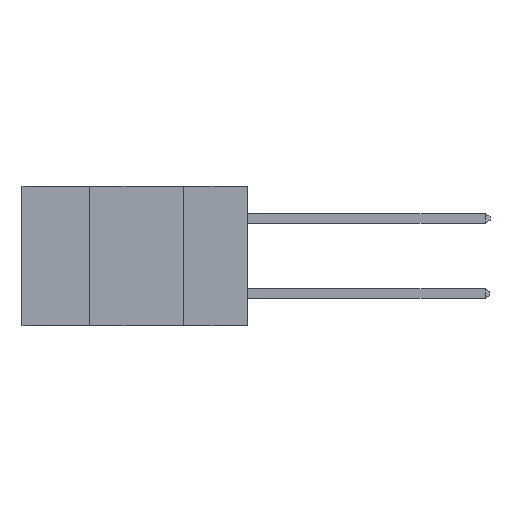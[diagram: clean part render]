
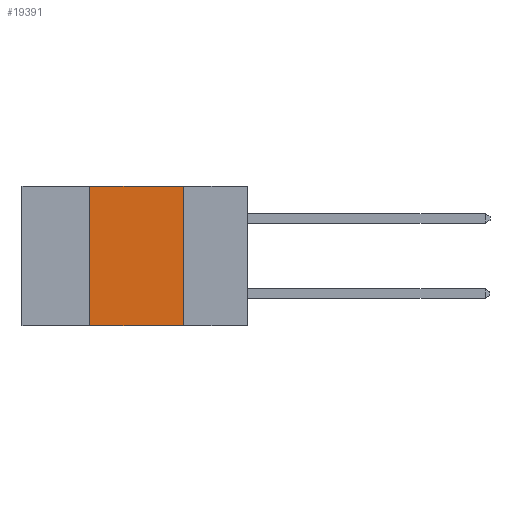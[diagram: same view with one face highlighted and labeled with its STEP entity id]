
A CAD part, left-side view. The second image highlights one B-rep face of the part: STEP entity #19391.
In plain terms, the highlighted planar face has unit normal (-1, 0, 0).
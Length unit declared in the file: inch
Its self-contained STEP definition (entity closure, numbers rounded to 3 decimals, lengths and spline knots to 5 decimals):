
#602 = LINE ( 'NONE', #23984, #11692 ) ;
#4492 = CARTESIAN_POINT ( 'NONE',  ( 0., 0.17, 0. ) ) ;
#5108 = VECTOR ( 'NONE', #9847, 39.37008 ) ;
#5384 = CARTESIAN_POINT ( 'NONE',  ( 0., 0.17, 0. ) ) ;
#6314 = CARTESIAN_POINT ( 'NONE',  ( 0., 0.6, 0. ) ) ;
#6433 = FACE_OUTER_BOUND ( 'NONE', #7102, .T. ) ;
#7102 = EDGE_LOOP ( 'NONE', ( #22584, #9074, #13600, #27208 ) ) ;
#7973 = DIRECTION ( 'NONE',  ( 0., 0., 1. ) ) ;
#8527 = DIRECTION ( 'NONE',  ( 1., 0., 0. ) ) ;
#9074 = ORIENTED_EDGE ( 'NONE', *, *, #26314, .F. ) ;
#9847 = DIRECTION ( 'NONE',  ( 0., 0., -1. ) ) ;
#10412 = LINE ( 'NONE', #19048, #15598 ) ;
#10803 = EDGE_CURVE ( 'NONE', #16067, #24062, #21349, .T. ) ;
#11113 = CARTESIAN_POINT ( 'NONE',  ( 0., 0.6, -0.37 ) ) ;
#11692 = VECTOR ( 'NONE', #26208, 39.37008 ) ;
#13186 = EDGE_CURVE ( 'NONE', #16067, #26387, #10412, .T. ) ;
#13600 = ORIENTED_EDGE ( 'NONE', *, *, #13186, .F. ) ;
#15598 = VECTOR ( 'NONE', #7973, 39.37008 ) ;
#16067 = VERTEX_POINT ( 'NONE', #17226 ) ;
#16096 = VECTOR ( 'NONE', #26679, 39.37008 ) ;
#17226 = CARTESIAN_POINT ( 'NONE',  ( 0., 0.42, -0.37 ) ) ;
#17527 = CARTESIAN_POINT ( 'NONE',  ( 0., 0.42, 0. ) ) ;
#18536 = EDGE_CURVE ( 'NONE', #22885, #24062, #22858, .T. ) ;
#19048 = CARTESIAN_POINT ( 'NONE',  ( 0., 0.42, 0. ) ) ;
#19391 = ADVANCED_FACE ( 'NONE', ( #6433 ), #19603, .F. ) ;
#19603 = PLANE ( 'NONE',  #24088 ) ;
#21349 = LINE ( 'NONE', #11113, #16096 ) ;
#22584 = ORIENTED_EDGE ( 'NONE', *, *, #18536, .F. ) ;
#22858 = LINE ( 'NONE', #5384, #5108 ) ;
#22885 = VERTEX_POINT ( 'NONE', #4492 ) ;
#23984 = CARTESIAN_POINT ( 'NONE',  ( 0., 0.6, 0. ) ) ;
#24062 = VERTEX_POINT ( 'NONE', #28195 ) ;
#24088 = AXIS2_PLACEMENT_3D ( 'NONE', #6314, #8527, #24109 ) ;
#24109 = DIRECTION ( 'NONE',  ( 0., 0., -1. ) ) ;
#26208 = DIRECTION ( 'NONE',  ( 0., -1., 0. ) ) ;
#26314 = EDGE_CURVE ( 'NONE', #26387, #22885, #602, .T. ) ;
#26387 = VERTEX_POINT ( 'NONE', #17527 ) ;
#26679 = DIRECTION ( 'NONE',  ( 0., -1., 0. ) ) ;
#27208 = ORIENTED_EDGE ( 'NONE', *, *, #10803, .T. ) ;
#28195 = CARTESIAN_POINT ( 'NONE',  ( 0., 0.17, -0.37 ) ) ;
